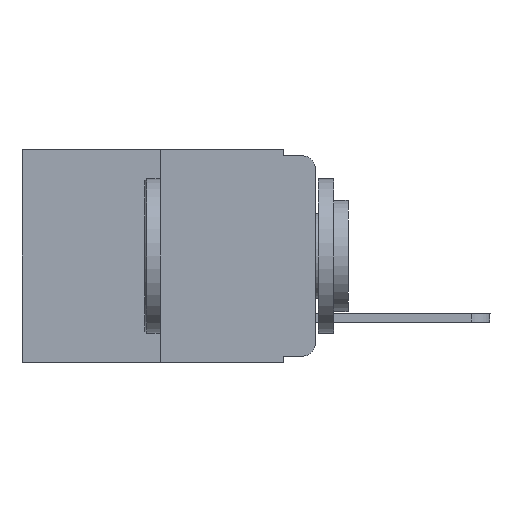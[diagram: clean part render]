
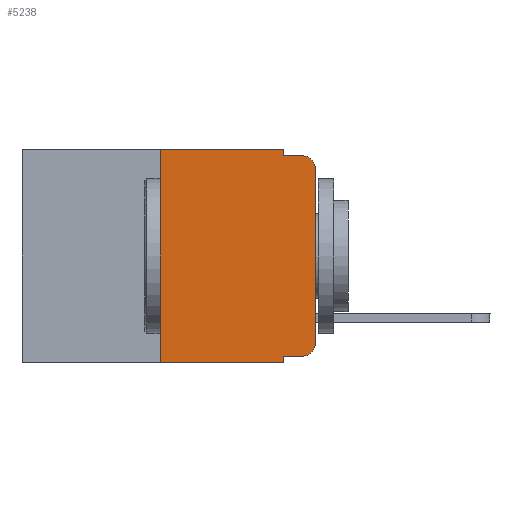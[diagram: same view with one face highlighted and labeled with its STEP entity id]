
A CAD part, left-side view. The second image highlights one B-rep face of the part: STEP entity #5238.
In plain terms, the highlighted planar face has unit normal (-1, 0, 0).
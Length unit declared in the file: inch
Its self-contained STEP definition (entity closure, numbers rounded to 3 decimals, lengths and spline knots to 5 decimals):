
#414 = CARTESIAN_POINT ( 'NONE',  ( 0., 0.051, -0.333 ) ) ;
#472 = LINE ( 'NONE', #5114, #7977 ) ;
#696 = LINE ( 'NONE', #7680, #1507 ) ;
#755 = CARTESIAN_POINT ( 'NONE',  ( 0., 0.473, 0. ) ) ;
#810 = VECTOR ( 'NONE', #2591, 39.37008 ) ;
#969 = EDGE_CURVE ( 'NONE', #3030, #14197, #10027, .T. ) ;
#982 = VECTOR ( 'NONE', #13177, 39.37008 ) ;
#1099 = DIRECTION ( 'NONE',  ( -1., 0., 0. ) ) ;
#1213 = EDGE_CURVE ( 'NONE', #3030, #7152, #11212, .T. ) ;
#1312 = CARTESIAN_POINT ( 'NONE',  ( 0., 0.051, -0.01 ) ) ;
#1434 = LINE ( 'NONE', #5086, #13133 ) ;
#1507 = VECTOR ( 'NONE', #14544, 39.37008 ) ;
#1626 = CARTESIAN_POINT ( 'NONE',  ( 0., 0.051, -0.343 ) ) ;
#2072 = CARTESIAN_POINT ( 'NONE',  ( 0., 0.473, 0. ) ) ;
#2509 = ORIENTED_EDGE ( 'NONE', *, *, #5823, .T. ) ;
#2591 = DIRECTION ( 'NONE',  ( 0., 0., 1. ) ) ;
#3002 = CARTESIAN_POINT ( 'NONE',  ( 0., 0.25, -0.343 ) ) ;
#3030 = VERTEX_POINT ( 'NONE', #3002 ) ;
#3221 = VECTOR ( 'NONE', #10255, 39.37008 ) ;
#3376 = VERTEX_POINT ( 'NONE', #11367 ) ;
#3595 = CIRCLE ( 'NONE', #11139, 0.02 ) ;
#4030 = CARTESIAN_POINT ( 'NONE',  ( 0., 0., 0. ) ) ;
#4032 = EDGE_CURVE ( 'NONE', #11170, #6990, #9525, .T. ) ;
#4076 = VERTEX_POINT ( 'NONE', #14477 ) ;
#4294 = CARTESIAN_POINT ( 'NONE',  ( 0., 0.473, -0.343 ) ) ;
#4650 = CIRCLE ( 'NONE', #9016, 0.02 ) ;
#4795 = ORIENTED_EDGE ( 'NONE', *, *, #969, .T. ) ;
#4801 = EDGE_CURVE ( 'NONE', #7152, #3376, #7602, .T. ) ;
#5086 = CARTESIAN_POINT ( 'NONE',  ( 0., 0.051, -0.333 ) ) ;
#5114 = CARTESIAN_POINT ( 'NONE',  ( 0., 0.051, 0. ) ) ;
#5238 = ADVANCED_FACE ( 'NONE', ( #5886 ), #10538, .F. ) ;
#5319 = ORIENTED_EDGE ( 'NONE', *, *, #15014, .T. ) ;
#5409 = EDGE_CURVE ( 'NONE', #3376, #10110, #696, .T. ) ;
#5659 = DIRECTION ( 'NONE',  ( 0., 0., -1. ) ) ;
#5823 = EDGE_CURVE ( 'NONE', #11465, #11170, #4650, .T. ) ;
#5886 = FACE_OUTER_BOUND ( 'NONE', #12227, .T. ) ;
#6001 = ORIENTED_EDGE ( 'NONE', *, *, #4032, .T. ) ;
#6184 = DIRECTION ( 'NONE',  ( 0., 0., -1. ) ) ;
#6939 = DIRECTION ( 'NONE',  ( 0., 0., -1. ) ) ;
#6990 = VERTEX_POINT ( 'NONE', #12842 ) ;
#7152 = VERTEX_POINT ( 'NONE', #13572 ) ;
#7602 = LINE ( 'NONE', #755, #3221 ) ;
#7680 = CARTESIAN_POINT ( 'NONE',  ( 0., 0.051, 0. ) ) ;
#7683 = DIRECTION ( 'NONE',  ( 0., 0., 1. ) ) ;
#7758 = EDGE_CURVE ( 'NONE', #10110, #4076, #12868, .T. ) ;
#7977 = VECTOR ( 'NONE', #6184, 39.37008 ) ;
#8036 = EDGE_CURVE ( 'NONE', #6990, #4076, #3595, .T. ) ;
#8274 = ORIENTED_EDGE ( 'NONE', *, *, #1213, .F. ) ;
#8748 = CARTESIAN_POINT ( 'NONE',  ( 0., 0.02, -0.03 ) ) ;
#8823 = CARTESIAN_POINT ( 'NONE',  ( 0., 0.25, 0. ) ) ;
#9016 = AXIS2_PLACEMENT_3D ( 'NONE', #9131, #1099, #6939 ) ;
#9131 = CARTESIAN_POINT ( 'NONE',  ( 0., 0.02, -0.313 ) ) ;
#9244 = AXIS2_PLACEMENT_3D ( 'NONE', #2072, #11372, #5659 ) ;
#9525 = LINE ( 'NONE', #4030, #810 ) ;
#9596 = CARTESIAN_POINT ( 'NONE',  ( 0., 0., -0.313 ) ) ;
#10027 = LINE ( 'NONE', #4294, #12948 ) ;
#10107 = VECTOR ( 'NONE', #7683, 39.37008 ) ;
#10110 = VERTEX_POINT ( 'NONE', #10534 ) ;
#10120 = CARTESIAN_POINT ( 'NONE',  ( 0., 0.02, -0.333 ) ) ;
#10255 = DIRECTION ( 'NONE',  ( 0., -1., 0. ) ) ;
#10534 = CARTESIAN_POINT ( 'NONE',  ( 0., 0.051, -0.01 ) ) ;
#10538 = PLANE ( 'NONE',  #9244 ) ;
#10806 = DIRECTION ( 'NONE',  ( 0., -1., 0. ) ) ;
#11139 = AXIS2_PLACEMENT_3D ( 'NONE', #8748, #13486, #12207 ) ;
#11170 = VERTEX_POINT ( 'NONE', #9596 ) ;
#11212 = LINE ( 'NONE', #8823, #10107 ) ;
#11259 = EDGE_CURVE ( 'NONE', #14143, #14197, #472, .T. ) ;
#11298 = ORIENTED_EDGE ( 'NONE', *, *, #4801, .F. ) ;
#11340 = ORIENTED_EDGE ( 'NONE', *, *, #7758, .F. ) ;
#11367 = CARTESIAN_POINT ( 'NONE',  ( 0., 0.051, 0. ) ) ;
#11372 = DIRECTION ( 'NONE',  ( 1., 0., 0. ) ) ;
#11465 = VERTEX_POINT ( 'NONE', #10120 ) ;
#11552 = ORIENTED_EDGE ( 'NONE', *, *, #11259, .F. ) ;
#12207 = DIRECTION ( 'NONE',  ( 0., 0., -1. ) ) ;
#12227 = EDGE_LOOP ( 'NONE', ( #6001, #14811, #11340, #12392, #11298, #8274, #4795, #11552, #5319, #2509 ) ) ;
#12392 = ORIENTED_EDGE ( 'NONE', *, *, #5409, .F. ) ;
#12842 = CARTESIAN_POINT ( 'NONE',  ( 0., 0., -0.03 ) ) ;
#12868 = LINE ( 'NONE', #1312, #982 ) ;
#12948 = VECTOR ( 'NONE', #14588, 39.37008 ) ;
#13133 = VECTOR ( 'NONE', #10806, 39.37008 ) ;
#13177 = DIRECTION ( 'NONE',  ( 0., -1., 0. ) ) ;
#13486 = DIRECTION ( 'NONE',  ( -1., 0., 0. ) ) ;
#13572 = CARTESIAN_POINT ( 'NONE',  ( 0., 0.25, 0. ) ) ;
#14143 = VERTEX_POINT ( 'NONE', #414 ) ;
#14197 = VERTEX_POINT ( 'NONE', #1626 ) ;
#14477 = CARTESIAN_POINT ( 'NONE',  ( 0., 0.02, -0.01 ) ) ;
#14544 = DIRECTION ( 'NONE',  ( 0., 0., -1. ) ) ;
#14588 = DIRECTION ( 'NONE',  ( 0., -1., 0. ) ) ;
#14811 = ORIENTED_EDGE ( 'NONE', *, *, #8036, .T. ) ;
#15014 = EDGE_CURVE ( 'NONE', #14143, #11465, #1434, .T. ) ;
